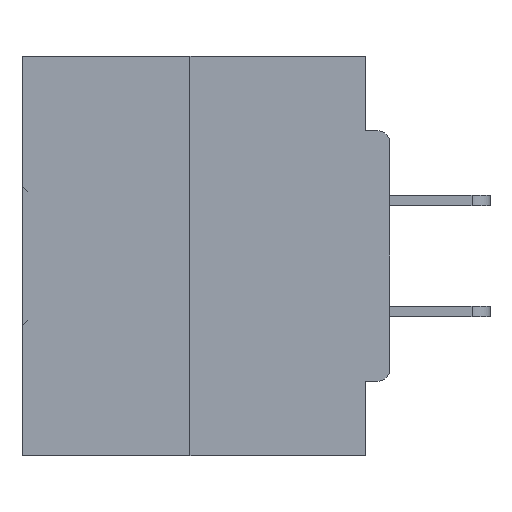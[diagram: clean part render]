
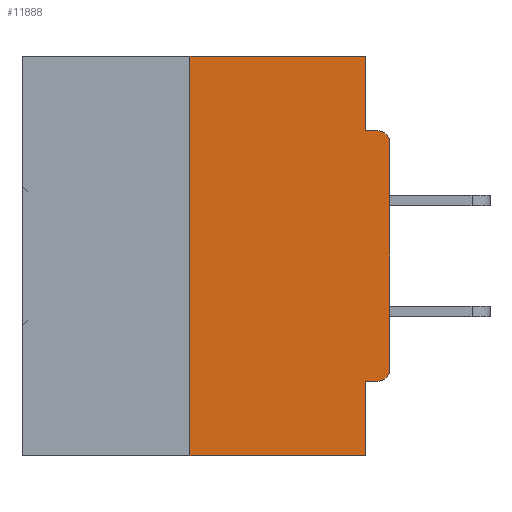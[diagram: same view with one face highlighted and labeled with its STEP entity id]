
A CAD part, left-side view. The second image highlights one B-rep face of the part: STEP entity #11888.
In plain terms, the highlighted planar face has unit normal (-1, 0, 0).
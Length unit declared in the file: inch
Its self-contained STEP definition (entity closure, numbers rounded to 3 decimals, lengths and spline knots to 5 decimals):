
#816 = ORIENTED_EDGE ( 'NONE', *, *, #41313, .F. ) ;
#1559 = LINE ( 'NONE', #8023, #4980 ) ;
#1785 = CARTESIAN_POINT ( 'NONE',  ( 0., 0.031, -0.4065 ) ) ;
#1836 = DIRECTION ( 'NONE',  ( 0., 0., 1. ) ) ;
#2826 = ORIENTED_EDGE ( 'NONE', *, *, #31453, .F. ) ;
#2845 = ORIENTED_EDGE ( 'NONE', *, *, #12179, .F. ) ;
#3074 = VERTEX_POINT ( 'NONE', #37487 ) ;
#3661 = DIRECTION ( 'NONE',  ( 0., 0., -1. ) ) ;
#4172 = VERTEX_POINT ( 'NONE', #41842 ) ;
#4643 = LINE ( 'NONE', #27056, #6353 ) ;
#4980 = VECTOR ( 'NONE', #40811, 39.37008 ) ;
#5303 = CARTESIAN_POINT ( 'NONE',  ( 0., 0.46, 0. ) ) ;
#5492 = CARTESIAN_POINT ( 'NONE',  ( 0., 0.25, 0. ) ) ;
#5982 = CARTESIAN_POINT ( 'NONE',  ( 0., 0., -0.4065 ) ) ;
#6108 = VERTEX_POINT ( 'NONE', #1785 ) ;
#6353 = VECTOR ( 'NONE', #9635, 39.37008 ) ;
#6476 = VERTEX_POINT ( 'NONE', #10233 ) ;
#6946 = ORIENTED_EDGE ( 'NONE', *, *, #21222, .F. ) ;
#7073 = CARTESIAN_POINT ( 'NONE',  ( 0., 0.031, -0.0935 ) ) ;
#7114 = CARTESIAN_POINT ( 'NONE',  ( 0., 0.015, -0.1085 ) ) ;
#7220 = VERTEX_POINT ( 'NONE', #25751 ) ;
#8023 = CARTESIAN_POINT ( 'NONE',  ( 0., 0.46, -0.5 ) ) ;
#8372 = LINE ( 'NONE', #27743, #12896 ) ;
#9303 = VERTEX_POINT ( 'NONE', #7073 ) ;
#9635 = DIRECTION ( 'NONE',  ( 0., 0., 1. ) ) ;
#10233 = CARTESIAN_POINT ( 'NONE',  ( 0., 0.031, -0.5 ) ) ;
#11888 = ADVANCED_FACE ( 'NONE', ( #45024 ), #38043, .F. ) ;
#12052 = CARTESIAN_POINT ( 'NONE',  ( 0., 0., -0.1085 ) ) ;
#12179 = EDGE_CURVE ( 'NONE', #30521, #7220, #21988, .T. ) ;
#12668 = VECTOR ( 'NONE', #1836, 39.37008 ) ;
#12896 = VECTOR ( 'NONE', #38119, 39.37008 ) ;
#16158 = CARTESIAN_POINT ( 'NONE',  ( 0., 0.031, 0. ) ) ;
#17276 = EDGE_CURVE ( 'NONE', #37664, #6476, #1559, .T. ) ;
#19087 = ORIENTED_EDGE ( 'NONE', *, *, #38089, .T. ) ;
#20101 = DIRECTION ( 'NONE',  ( 0., 1., 0. ) ) ;
#21222 = EDGE_CURVE ( 'NONE', #37664, #30521, #43525, .T. ) ;
#21581 = DIRECTION ( 'NONE',  ( -1., 0., 0. ) ) ;
#21851 = CARTESIAN_POINT ( 'NONE',  ( 0., 0.46, 0. ) ) ;
#21964 = CARTESIAN_POINT ( 'NONE',  ( 0., 0.25, -0.5 ) ) ;
#21988 = LINE ( 'NONE', #5303, #23687 ) ;
#23687 = VECTOR ( 'NONE', #30391, 39.37008 ) ;
#23950 = CARTESIAN_POINT ( 'NONE',  ( 0., 0.031, -0.5 ) ) ;
#25024 = DIRECTION ( 'NONE',  ( 1., 0., 0. ) ) ;
#25169 = DIRECTION ( 'NONE',  ( 0., 0., -1. ) ) ;
#25549 = AXIS2_PLACEMENT_3D ( 'NONE', #44443, #31454, #30181 ) ;
#25663 = AXIS2_PLACEMENT_3D ( 'NONE', #21851, #25024, #25169 ) ;
#25722 = VERTEX_POINT ( 'NONE', #30292 ) ;
#25751 = CARTESIAN_POINT ( 'NONE',  ( 0., 0.031, 0. ) ) ;
#26683 = LINE ( 'NONE', #23950, #44609 ) ;
#27056 = CARTESIAN_POINT ( 'NONE',  ( 0., 0., 0. ) ) ;
#27743 = CARTESIAN_POINT ( 'NONE',  ( 0., 0., -0.0935 ) ) ;
#27784 = LINE ( 'NONE', #5982, #30564 ) ;
#29242 = ORIENTED_EDGE ( 'NONE', *, *, #44699, .F. ) ;
#30181 = DIRECTION ( 'NONE',  ( 0., 0., -1. ) ) ;
#30266 = DIRECTION ( 'NONE',  ( 0., 0., -1. ) ) ;
#30292 = CARTESIAN_POINT ( 'NONE',  ( 0., 0.015, -0.4065 ) ) ;
#30391 = DIRECTION ( 'NONE',  ( 0., -1., 0. ) ) ;
#30465 = LINE ( 'NONE', #16158, #46156 ) ;
#30521 = VERTEX_POINT ( 'NONE', #37397 ) ;
#30564 = VECTOR ( 'NONE', #20101, 39.37008 ) ;
#31043 = EDGE_CURVE ( 'NONE', #4172, #46135, #4643, .T. ) ;
#31453 = EDGE_CURVE ( 'NONE', #7220, #9303, #30465, .T. ) ;
#31454 = DIRECTION ( 'NONE',  ( -1., 0., 0. ) ) ;
#34861 = AXIS2_PLACEMENT_3D ( 'NONE', #7114, #21581, #3661 ) ;
#36594 = CIRCLE ( 'NONE', #34861, 0.015 ) ;
#37397 = CARTESIAN_POINT ( 'NONE',  ( 0., 0.25, 0. ) ) ;
#37487 = CARTESIAN_POINT ( 'NONE',  ( 0., 0.015, -0.0935 ) ) ;
#37664 = VERTEX_POINT ( 'NONE', #21964 ) ;
#37829 = ORIENTED_EDGE ( 'NONE', *, *, #31043, .T. ) ;
#38043 = PLANE ( 'NONE',  #25663 ) ;
#38089 = EDGE_CURVE ( 'NONE', #25722, #4172, #41832, .T. ) ;
#38119 = DIRECTION ( 'NONE',  ( 0., -1., 0. ) ) ;
#38386 = DIRECTION ( 'NONE',  ( 0., 0., -1. ) ) ;
#39070 = EDGE_CURVE ( 'NONE', #46135, #3074, #36594, .T. ) ;
#40523 = ORIENTED_EDGE ( 'NONE', *, *, #39070, .T. ) ;
#40811 = DIRECTION ( 'NONE',  ( 0., -1., 0. ) ) ;
#41313 = EDGE_CURVE ( 'NONE', #9303, #3074, #8372, .T. ) ;
#41832 = CIRCLE ( 'NONE', #25549, 0.015 ) ;
#41842 = CARTESIAN_POINT ( 'NONE',  ( 0., 0., -0.3915 ) ) ;
#42503 = EDGE_LOOP ( 'NONE', ( #2845, #6946, #46218, #43254, #29242, #19087, #37829, #40523, #816, #2826 ) ) ;
#43254 = ORIENTED_EDGE ( 'NONE', *, *, #44111, .F. ) ;
#43525 = LINE ( 'NONE', #5492, #12668 ) ;
#44111 = EDGE_CURVE ( 'NONE', #6108, #6476, #26683, .T. ) ;
#44443 = CARTESIAN_POINT ( 'NONE',  ( 0., 0.015, -0.3915 ) ) ;
#44609 = VECTOR ( 'NONE', #38386, 39.37008 ) ;
#44699 = EDGE_CURVE ( 'NONE', #25722, #6108, #27784, .T. ) ;
#45024 = FACE_OUTER_BOUND ( 'NONE', #42503, .T. ) ;
#46135 = VERTEX_POINT ( 'NONE', #12052 ) ;
#46156 = VECTOR ( 'NONE', #30266, 39.37008 ) ;
#46218 = ORIENTED_EDGE ( 'NONE', *, *, #17276, .T. ) ;
